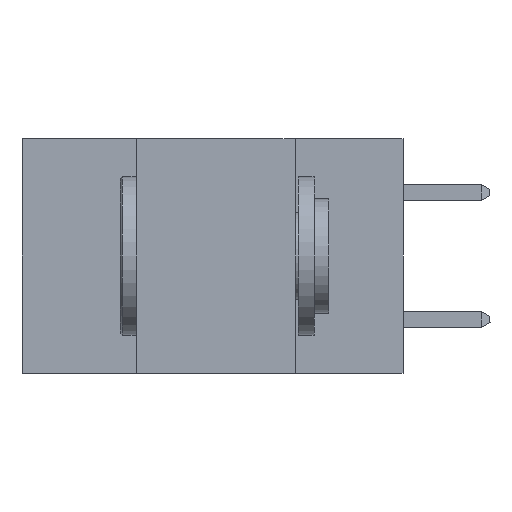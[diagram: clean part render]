
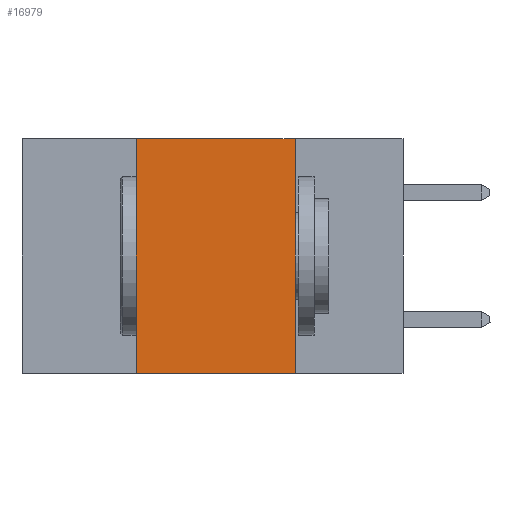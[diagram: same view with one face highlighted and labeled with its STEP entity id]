
A CAD part, left-side view. The second image highlights one B-rep face of the part: STEP entity #16979.
In plain terms, the highlighted planar face has unit normal (-1, 0, 0).
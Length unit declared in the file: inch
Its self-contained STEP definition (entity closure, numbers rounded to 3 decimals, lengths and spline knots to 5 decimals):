
#85 = VERTEX_POINT ( 'NONE', #341 ) ;
#307 = DIRECTION ( 'NONE',  ( 0., 0., 1. ) ) ;
#341 = CARTESIAN_POINT ( 'NONE',  ( 0., 0.42, 0. ) ) ;
#875 = CARTESIAN_POINT ( 'NONE',  ( 0., 0.42, -0.37 ) ) ;
#1019 = DIRECTION ( 'NONE',  ( 0., 0., -1. ) ) ;
#1279 = CARTESIAN_POINT ( 'NONE',  ( 0., 0.17, -0.37 ) ) ;
#1816 = VECTOR ( 'NONE', #1019, 39.37008 ) ;
#2232 = VERTEX_POINT ( 'NONE', #13636 ) ;
#2908 = VERTEX_POINT ( 'NONE', #1279 ) ;
#3909 = ORIENTED_EDGE ( 'NONE', *, *, #12723, .F. ) ;
#4537 = ORIENTED_EDGE ( 'NONE', *, *, #14384, .F. ) ;
#4784 = VECTOR ( 'NONE', #307, 39.37008 ) ;
#5699 = VECTOR ( 'NONE', #19459, 39.37008 ) ;
#7298 = DIRECTION ( 'NONE',  ( 0., -1., 0. ) ) ;
#8407 = CARTESIAN_POINT ( 'NONE',  ( 0., 0.6, 0. ) ) ;
#9895 = LINE ( 'NONE', #10611, #13661 ) ;
#10000 = PLANE ( 'NONE',  #12932 ) ;
#10067 = DIRECTION ( 'NONE',  ( 0., 0., -1. ) ) ;
#10611 = CARTESIAN_POINT ( 'NONE',  ( 0., 0.6, -0.37 ) ) ;
#11202 = LINE ( 'NONE', #20789, #1816 ) ;
#11323 = CARTESIAN_POINT ( 'NONE',  ( 0., 0.6, 0. ) ) ;
#11920 = ORIENTED_EDGE ( 'NONE', *, *, #16852, .F. ) ;
#11941 = CARTESIAN_POINT ( 'NONE',  ( 0., 0.42, 0. ) ) ;
#11982 = EDGE_LOOP ( 'NONE', ( #4537, #11920, #3909, #16817 ) ) ;
#12723 = EDGE_CURVE ( 'NONE', #14349, #85, #12998, .T. ) ;
#12932 = AXIS2_PLACEMENT_3D ( 'NONE', #8407, #19800, #10067 ) ;
#12998 = LINE ( 'NONE', #11941, #4784 ) ;
#13636 = CARTESIAN_POINT ( 'NONE',  ( 0., 0.17, 0. ) ) ;
#13661 = VECTOR ( 'NONE', #7298, 39.37008 ) ;
#14349 = VERTEX_POINT ( 'NONE', #875 ) ;
#14384 = EDGE_CURVE ( 'NONE', #2232, #2908, #11202, .T. ) ;
#15458 = EDGE_CURVE ( 'NONE', #14349, #2908, #9895, .T. ) ;
#16817 = ORIENTED_EDGE ( 'NONE', *, *, #15458, .T. ) ;
#16852 = EDGE_CURVE ( 'NONE', #85, #2232, #18787, .T. ) ;
#16979 = ADVANCED_FACE ( 'NONE', ( #20569 ), #10000, .F. ) ;
#18787 = LINE ( 'NONE', #11323, #5699 ) ;
#19459 = DIRECTION ( 'NONE',  ( 0., -1., 0. ) ) ;
#19800 = DIRECTION ( 'NONE',  ( 1., 0., 0. ) ) ;
#20569 = FACE_OUTER_BOUND ( 'NONE', #11982, .T. ) ;
#20789 = CARTESIAN_POINT ( 'NONE',  ( 0., 0.17, 0. ) ) ;
